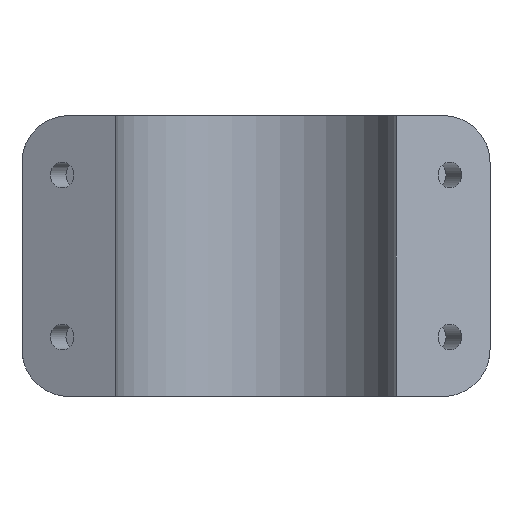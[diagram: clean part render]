
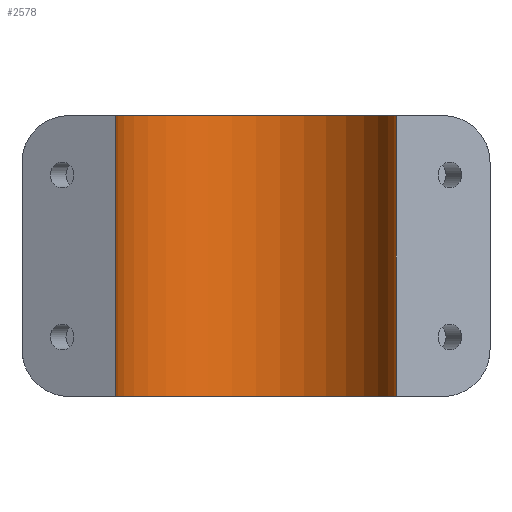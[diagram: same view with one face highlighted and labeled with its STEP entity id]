
A CAD part, left-side view. The second image highlights one B-rep face of the part: STEP entity #2578.
In plain terms, the highlighted cylindrical face has radius 19.05 mm (diameter 38.1 mm), a partial arc.
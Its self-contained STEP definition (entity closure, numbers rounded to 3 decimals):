
#38 = LINE ( 'NONE', #2224, #2264 ) ;
#109 = VERTEX_POINT ( 'NONE', #1237 ) ;
#153 = CARTESIAN_POINT ( 'NONE',  ( -50.8, -19.05, 12.7 ) ) ;
#194 = AXIS2_PLACEMENT_3D ( 'NONE', #349, #1842, #574 ) ;
#300 = CARTESIAN_POINT ( 'NONE',  ( -50.8, -19.05, -129.548 ) ) ;
#349 = CARTESIAN_POINT ( 'NONE',  ( -50.8, 0., 12.7 ) ) ;
#354 = EDGE_CURVE ( 'NONE', #2233, #992, #1566, .T. ) ;
#447 = ORIENTED_EDGE ( 'NONE', *, *, #2216, .F. ) ;
#472 = AXIS2_PLACEMENT_3D ( 'NONE', #1862, #584, #2075 ) ;
#479 = VERTEX_POINT ( 'NONE', #1623 ) ;
#503 = EDGE_CURVE ( 'NONE', #2233, #479, #2234, .T. ) ;
#512 = DIRECTION ( 'NONE',  ( 0., 0., -1. ) ) ;
#519 = EDGE_LOOP ( 'NONE', ( #1074, #1071, #447, #1978 ) ) ;
#574 = DIRECTION ( 'NONE',  ( 1., 0., 0. ) ) ;
#584 = DIRECTION ( 'NONE',  ( 0., 0., 1. ) ) ;
#634 = CARTESIAN_POINT ( 'NONE',  ( -50.8, -19.05, -25.4 ) ) ;
#851 = DIRECTION ( 'NONE',  ( 1., 0., 0. ) ) ;
#950 = AXIS2_PLACEMENT_3D ( 'NONE', #2343, #1491, #851 ) ;
#958 = DIRECTION ( 'NONE',  ( 0., 0., -1. ) ) ;
#992 = VERTEX_POINT ( 'NONE', #634 ) ;
#1071 = ORIENTED_EDGE ( 'NONE', *, *, #1162, .T. ) ;
#1074 = ORIENTED_EDGE ( 'NONE', *, *, #503, .T. ) ;
#1093 = CIRCLE ( 'NONE', #472, 19.05 ) ;
#1162 = EDGE_CURVE ( 'NONE', #479, #109, #38, .T. ) ;
#1237 = CARTESIAN_POINT ( 'NONE',  ( -50.8, 19.05, -25.4 ) ) ;
#1491 = DIRECTION ( 'NONE',  ( 0., 0., 1. ) ) ;
#1566 = LINE ( 'NONE', #300, #2590 ) ;
#1623 = CARTESIAN_POINT ( 'NONE',  ( -50.8, 19.05, 12.7 ) ) ;
#1842 = DIRECTION ( 'NONE',  ( 0., 0., 1. ) ) ;
#1862 = CARTESIAN_POINT ( 'NONE',  ( -50.8, 0., -25.4 ) ) ;
#1978 = ORIENTED_EDGE ( 'NONE', *, *, #354, .F. ) ;
#2075 = DIRECTION ( 'NONE',  ( -1., 0., 0. ) ) ;
#2216 = EDGE_CURVE ( 'NONE', #992, #109, #1093, .T. ) ;
#2224 = CARTESIAN_POINT ( 'NONE',  ( -50.8, 19.05, -129.548 ) ) ;
#2233 = VERTEX_POINT ( 'NONE', #153 ) ;
#2234 = CIRCLE ( 'NONE', #194, 19.05 ) ;
#2264 = VECTOR ( 'NONE', #958, 1000. ) ;
#2293 = CYLINDRICAL_SURFACE ( 'NONE', #950, 19.05 ) ;
#2343 = CARTESIAN_POINT ( 'NONE',  ( -50.8, 0., -129.548 ) ) ;
#2354 = FACE_OUTER_BOUND ( 'NONE', #519, .T. ) ;
#2578 = ADVANCED_FACE ( 'NONE', ( #2354 ), #2293, .F. ) ;
#2590 = VECTOR ( 'NONE', #512, 1000. ) ;
